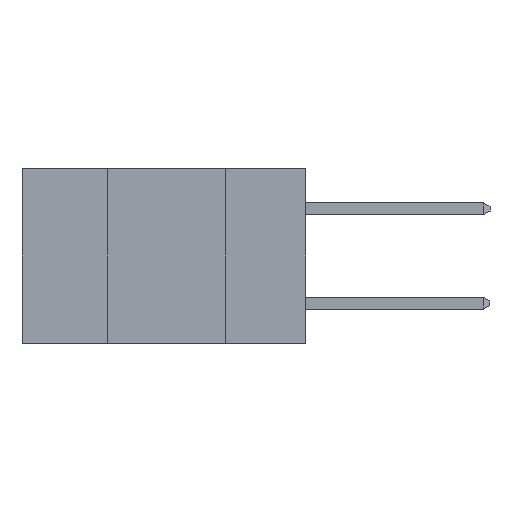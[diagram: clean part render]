
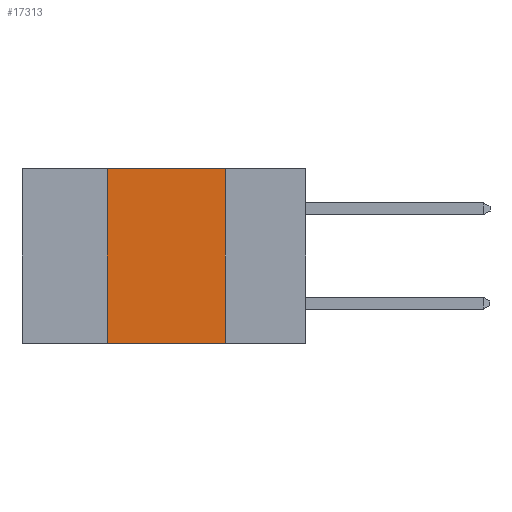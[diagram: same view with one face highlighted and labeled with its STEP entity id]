
A CAD part, left-side view. The second image highlights one B-rep face of the part: STEP entity #17313.
In plain terms, the highlighted planar face has unit normal (-1, 0, 0).
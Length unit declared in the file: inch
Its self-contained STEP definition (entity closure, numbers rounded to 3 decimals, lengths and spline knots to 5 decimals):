
#992 = CARTESIAN_POINT ( 'NONE',  ( 0., 0.42, 0. ) ) ;
#1057 = CARTESIAN_POINT ( 'NONE',  ( 0., 0.6, 0. ) ) ;
#1133 = DIRECTION ( 'NONE',  ( 1., 0., 0. ) ) ;
#2020 = VERTEX_POINT ( 'NONE', #8773 ) ;
#2737 = CARTESIAN_POINT ( 'NONE',  ( 0., 0.6, -0.37 ) ) ;
#3017 = LINE ( 'NONE', #2737, #6526 ) ;
#3176 = ORIENTED_EDGE ( 'NONE', *, *, #10084, .T. ) ;
#3720 = DIRECTION ( 'NONE',  ( 0., -1., 0. ) ) ;
#5222 = ORIENTED_EDGE ( 'NONE', *, *, #11452, .F. ) ;
#6526 = VECTOR ( 'NONE', #16099, 39.37008 ) ;
#6527 = LINE ( 'NONE', #14084, #13929 ) ;
#8333 = CARTESIAN_POINT ( 'NONE',  ( 0., 0.42, 0. ) ) ;
#8773 = CARTESIAN_POINT ( 'NONE',  ( 0., 0.42, -0.37 ) ) ;
#10084 = EDGE_CURVE ( 'NONE', #2020, #10883, #3017, .T. ) ;
#10086 = PLANE ( 'NONE',  #12494 ) ;
#10261 = ORIENTED_EDGE ( 'NONE', *, *, #16502, .F. ) ;
#10325 = LINE ( 'NONE', #8333, #10787 ) ;
#10719 = VERTEX_POINT ( 'NONE', #14073 ) ;
#10787 = VECTOR ( 'NONE', #17137, 39.37008 ) ;
#10883 = VERTEX_POINT ( 'NONE', #11442 ) ;
#11282 = CARTESIAN_POINT ( 'NONE',  ( 0., 0.17, 0. ) ) ;
#11418 = VECTOR ( 'NONE', #12797, 39.37008 ) ;
#11442 = CARTESIAN_POINT ( 'NONE',  ( 0., 0.17, -0.37 ) ) ;
#11452 = EDGE_CURVE ( 'NONE', #10719, #10883, #16750, .T. ) ;
#11564 = DIRECTION ( 'NONE',  ( 0., 0., -1. ) ) ;
#12494 = AXIS2_PLACEMENT_3D ( 'NONE', #1057, #1133, #11564 ) ;
#12797 = DIRECTION ( 'NONE',  ( 0., 0., -1. ) ) ;
#13319 = EDGE_CURVE ( 'NONE', #19087, #10719, #6527, .T. ) ;
#13362 = EDGE_LOOP ( 'NONE', ( #5222, #15616, #10261, #3176 ) ) ;
#13929 = VECTOR ( 'NONE', #3720, 39.37008 ) ;
#14073 = CARTESIAN_POINT ( 'NONE',  ( 0., 0.17, 0. ) ) ;
#14084 = CARTESIAN_POINT ( 'NONE',  ( 0., 0.6, 0. ) ) ;
#15616 = ORIENTED_EDGE ( 'NONE', *, *, #13319, .F. ) ;
#16099 = DIRECTION ( 'NONE',  ( 0., -1., 0. ) ) ;
#16482 = FACE_OUTER_BOUND ( 'NONE', #13362, .T. ) ;
#16502 = EDGE_CURVE ( 'NONE', #2020, #19087, #10325, .T. ) ;
#16750 = LINE ( 'NONE', #11282, #11418 ) ;
#17137 = DIRECTION ( 'NONE',  ( 0., 0., 1. ) ) ;
#17313 = ADVANCED_FACE ( 'NONE', ( #16482 ), #10086, .F. ) ;
#19087 = VERTEX_POINT ( 'NONE', #992 ) ;
